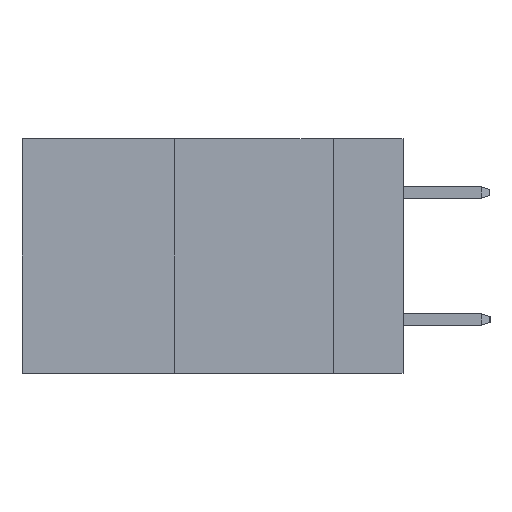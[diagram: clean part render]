
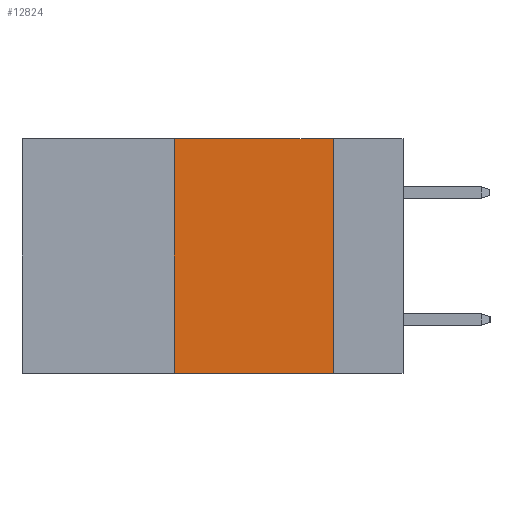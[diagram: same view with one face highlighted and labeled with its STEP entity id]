
A CAD part, left-side view. The second image highlights one B-rep face of the part: STEP entity #12824.
In plain terms, the highlighted planar face has unit normal (-1, 0, 0).
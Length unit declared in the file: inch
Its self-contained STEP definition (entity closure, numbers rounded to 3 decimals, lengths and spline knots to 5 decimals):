
#519 = DIRECTION ( 'NONE',  ( 0., -1., 0. ) ) ;
#566 = LINE ( 'NONE', #5207, #6869 ) ;
#695 = VERTEX_POINT ( 'NONE', #15015 ) ;
#882 = EDGE_LOOP ( 'NONE', ( #1371, #14986, #4750, #14029 ) ) ;
#1371 = ORIENTED_EDGE ( 'NONE', *, *, #13511, .F. ) ;
#1800 = VECTOR ( 'NONE', #519, 39.37008 ) ;
#1989 = LINE ( 'NONE', #4764, #1800 ) ;
#2179 = VECTOR ( 'NONE', #3068, 39.37008 ) ;
#3068 = DIRECTION ( 'NONE',  ( 0., 0., 1. ) ) ;
#3072 = PLANE ( 'NONE',  #10957 ) ;
#4270 = CARTESIAN_POINT ( 'NONE',  ( 0., 0.6, 0. ) ) ;
#4483 = CARTESIAN_POINT ( 'NONE',  ( 0., 0.6, 0. ) ) ;
#4750 = ORIENTED_EDGE ( 'NONE', *, *, #17940, .F. ) ;
#4764 = CARTESIAN_POINT ( 'NONE',  ( 0., 0.6, -0.37 ) ) ;
#5207 = CARTESIAN_POINT ( 'NONE',  ( 0., 0.11, 0. ) ) ;
#6869 = VECTOR ( 'NONE', #18662, 39.37008 ) ;
#7244 = DIRECTION ( 'NONE',  ( 0., 0., -1. ) ) ;
#8985 = VERTEX_POINT ( 'NONE', #12576 ) ;
#10098 = CARTESIAN_POINT ( 'NONE',  ( 0., 0.11, -0.37 ) ) ;
#10434 = CARTESIAN_POINT ( 'NONE',  ( 0., 0.36, -0.37 ) ) ;
#10520 = DIRECTION ( 'NONE',  ( 0., -1., 0. ) ) ;
#10957 = AXIS2_PLACEMENT_3D ( 'NONE', #4270, #11972, #7244 ) ;
#11017 = VECTOR ( 'NONE', #10520, 39.37008 ) ;
#11972 = DIRECTION ( 'NONE',  ( 1., 0., 0. ) ) ;
#12343 = VERTEX_POINT ( 'NONE', #10434 ) ;
#12576 = CARTESIAN_POINT ( 'NONE',  ( 0., 0.11, 0. ) ) ;
#12824 = ADVANCED_FACE ( 'NONE', ( #13569 ), #3072, .F. ) ;
#12953 = EDGE_CURVE ( 'NONE', #12343, #13208, #1989, .T. ) ;
#13208 = VERTEX_POINT ( 'NONE', #10098 ) ;
#13511 = EDGE_CURVE ( 'NONE', #8985, #13208, #566, .T. ) ;
#13569 = FACE_OUTER_BOUND ( 'NONE', #882, .T. ) ;
#14029 = ORIENTED_EDGE ( 'NONE', *, *, #12953, .T. ) ;
#14848 = CARTESIAN_POINT ( 'NONE',  ( 0., 0.36, 0. ) ) ;
#14986 = ORIENTED_EDGE ( 'NONE', *, *, #19336, .F. ) ;
#15015 = CARTESIAN_POINT ( 'NONE',  ( 0., 0.36, 0. ) ) ;
#17940 = EDGE_CURVE ( 'NONE', #12343, #695, #19405, .T. ) ;
#18662 = DIRECTION ( 'NONE',  ( 0., 0., -1. ) ) ;
#19327 = LINE ( 'NONE', #4483, #11017 ) ;
#19336 = EDGE_CURVE ( 'NONE', #695, #8985, #19327, .T. ) ;
#19405 = LINE ( 'NONE', #14848, #2179 ) ;
